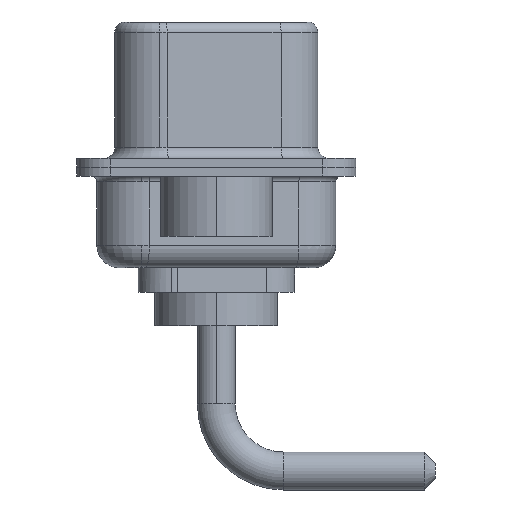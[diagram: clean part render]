
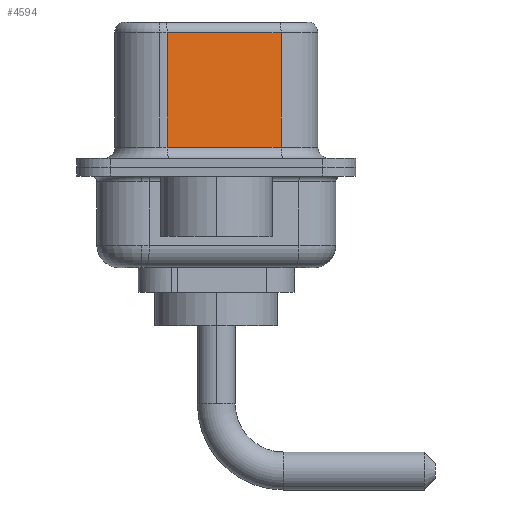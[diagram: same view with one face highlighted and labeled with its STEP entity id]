
A CAD part, left-side view. The second image highlights one B-rep face of the part: STEP entity #4594.
In plain terms, the highlighted planar face has unit normal (-0.985, -0.174, 0).
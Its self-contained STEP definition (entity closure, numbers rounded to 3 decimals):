
#101 = CARTESIAN_POINT ( 'NONE',  ( 4.555, -2.897, 6.52 ) ) ;
#380 = DIRECTION ( 'NONE',  ( 0.985, 0.174, 0. ) ) ;
#541 = DIRECTION ( 'NONE',  ( 0., 0., -1. ) ) ;
#694 = CARTESIAN_POINT ( 'NONE',  ( 3.655, 2.203, 6.02 ) ) ;
#855 = CARTESIAN_POINT ( 'NONE',  ( 4.555, -2.897, 0.9 ) ) ;
#884 = ORIENTED_EDGE ( 'NONE', *, *, #4375, .T. ) ;
#1567 = FACE_OUTER_BOUND ( 'NONE', #7099, .T. ) ;
#1638 = DIRECTION ( 'NONE',  ( -0.174, 0.985, 0. ) ) ;
#2354 = VERTEX_POINT ( 'NONE', #15158 ) ;
#2622 = LINE ( 'NONE', #13611, #9807 ) ;
#3020 = AXIS2_PLACEMENT_3D ( 'NONE', #4107, #380, #1638 ) ;
#3584 = DIRECTION ( 'NONE',  ( 0., 0., -1. ) ) ;
#4107 = CARTESIAN_POINT ( 'NONE',  ( 4.555, -2.897, 6.52 ) ) ;
#4375 = EDGE_CURVE ( 'NONE', #2354, #6105, #15739, .T. ) ;
#4475 = ORIENTED_EDGE ( 'NONE', *, *, #11844, .T. ) ;
#4594 = ADVANCED_FACE ( 'NONE', ( #1567 ), #12626, .F. ) ;
#4712 = ORIENTED_EDGE ( 'NONE', *, *, #15106, .F. ) ;
#4780 = LINE ( 'NONE', #101, #5828 ) ;
#4827 = CARTESIAN_POINT ( 'NONE',  ( 4.555, -2.897, 0.9 ) ) ;
#5068 = DIRECTION ( 'NONE',  ( 0.174, -0.985, 0. ) ) ;
#5828 = VECTOR ( 'NONE', #3584, 1000. ) ;
#6105 = VERTEX_POINT ( 'NONE', #855 ) ;
#6136 = CARTESIAN_POINT ( 'NONE',  ( 4.555, -2.897, 6.02 ) ) ;
#6586 = LINE ( 'NONE', #7553, #8045 ) ;
#7099 = EDGE_LOOP ( 'NONE', ( #4712, #11693, #4475, #884 ) ) ;
#7553 = CARTESIAN_POINT ( 'NONE',  ( 3.655, 2.203, 6.52 ) ) ;
#7624 = VECTOR ( 'NONE', #5068, 1000. ) ;
#8045 = VECTOR ( 'NONE', #541, 1000. ) ;
#9807 = VECTOR ( 'NONE', #13381, 1000. ) ;
#10296 = EDGE_CURVE ( 'NONE', #10356, #13365, #2622, .T. ) ;
#10356 = VERTEX_POINT ( 'NONE', #6136 ) ;
#11693 = ORIENTED_EDGE ( 'NONE', *, *, #10296, .T. ) ;
#11844 = EDGE_CURVE ( 'NONE', #13365, #2354, #6586, .T. ) ;
#12626 = PLANE ( 'NONE',  #3020 ) ;
#13365 = VERTEX_POINT ( 'NONE', #694 ) ;
#13381 = DIRECTION ( 'NONE',  ( -0.174, 0.985, 0. ) ) ;
#13611 = CARTESIAN_POINT ( 'NONE',  ( 4.555, -2.897, 6.02 ) ) ;
#15106 = EDGE_CURVE ( 'NONE', #10356, #6105, #4780, .T. ) ;
#15158 = CARTESIAN_POINT ( 'NONE',  ( 3.655, 2.203, 0.9 ) ) ;
#15739 = LINE ( 'NONE', #4827, #7624 ) ;
